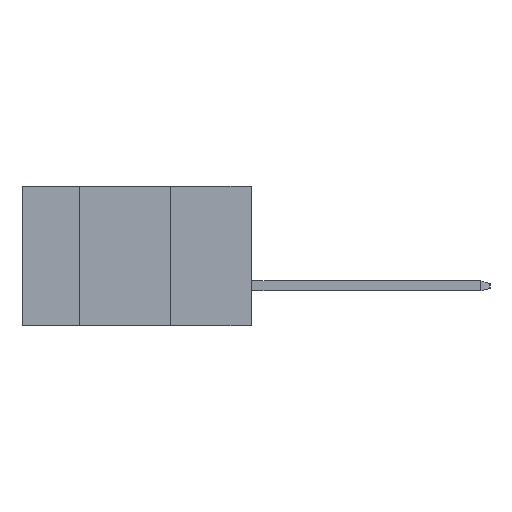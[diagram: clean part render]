
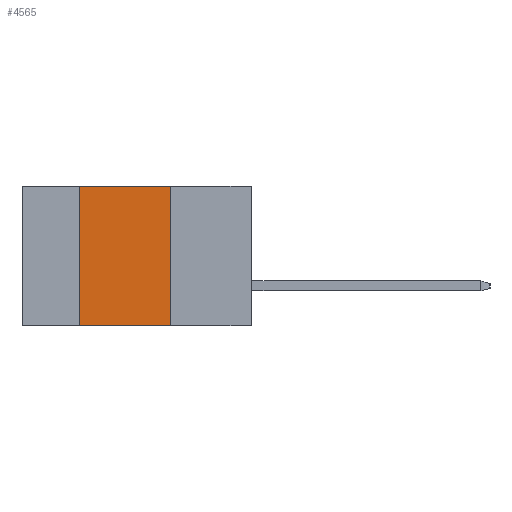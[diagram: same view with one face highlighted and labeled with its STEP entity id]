
A CAD part, left-side view. The second image highlights one B-rep face of the part: STEP entity #4565.
In plain terms, the highlighted planar face has unit normal (-1, 0, 0).
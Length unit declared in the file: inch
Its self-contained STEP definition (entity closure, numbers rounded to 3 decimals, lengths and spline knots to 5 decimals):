
#315 = EDGE_CURVE ( 'NONE', #5962, #707, #1120, .T. ) ;
#588 = CARTESIAN_POINT ( 'NONE',  ( 0., 0.54, -0.437 ) ) ;
#688 = CARTESIAN_POINT ( 'NONE',  ( 0., 0.72, 0. ) ) ;
#707 = VERTEX_POINT ( 'NONE', #6120 ) ;
#947 = ORIENTED_EDGE ( 'NONE', *, *, #7936, .T. ) ;
#1120 = LINE ( 'NONE', #6609, #1316 ) ;
#1316 = VECTOR ( 'NONE', #9772, 39.37008 ) ;
#1499 = ORIENTED_EDGE ( 'NONE', *, *, #315, .F. ) ;
#1582 = EDGE_LOOP ( 'NONE', ( #1499, #2919, #4034, #947 ) ) ;
#2122 = FACE_OUTER_BOUND ( 'NONE', #1582, .T. ) ;
#2214 = VECTOR ( 'NONE', #7254, 39.37008 ) ;
#2231 = DIRECTION ( 'NONE',  ( 1., 0., 0. ) ) ;
#2919 = ORIENTED_EDGE ( 'NONE', *, *, #5681, .F. ) ;
#3491 = AXIS2_PLACEMENT_3D ( 'NONE', #688, #2231, #10008 ) ;
#3810 = DIRECTION ( 'NONE',  ( 0., 0., 1. ) ) ;
#3975 = VERTEX_POINT ( 'NONE', #6569 ) ;
#4034 = ORIENTED_EDGE ( 'NONE', *, *, #6354, .F. ) ;
#4361 = CARTESIAN_POINT ( 'NONE',  ( 0., 0.72, -0.437 ) ) ;
#4501 = CARTESIAN_POINT ( 'NONE',  ( 0., 0.254, 0. ) ) ;
#4565 = ADVANCED_FACE ( 'NONE', ( #2122 ), #8394, .F. ) ;
#4643 = VECTOR ( 'NONE', #8728, 39.37008 ) ;
#4824 = CARTESIAN_POINT ( 'NONE',  ( 0., 0.72, 0. ) ) ;
#5681 = EDGE_CURVE ( 'NONE', #7654, #5962, #8578, .T. ) ;
#5962 = VERTEX_POINT ( 'NONE', #4501 ) ;
#6120 = CARTESIAN_POINT ( 'NONE',  ( 0., 0.254, -0.437 ) ) ;
#6190 = LINE ( 'NONE', #4361, #2214 ) ;
#6354 = EDGE_CURVE ( 'NONE', #3975, #7654, #9272, .T. ) ;
#6569 = CARTESIAN_POINT ( 'NONE',  ( 0., 0.54, -0.437 ) ) ;
#6609 = CARTESIAN_POINT ( 'NONE',  ( 0., 0.254, -0.437 ) ) ;
#7254 = DIRECTION ( 'NONE',  ( 0., -1., 0. ) ) ;
#7654 = VERTEX_POINT ( 'NONE', #8247 ) ;
#7936 = EDGE_CURVE ( 'NONE', #3975, #707, #6190, .T. ) ;
#8247 = CARTESIAN_POINT ( 'NONE',  ( 0., 0.54, 0. ) ) ;
#8394 = PLANE ( 'NONE',  #3491 ) ;
#8578 = LINE ( 'NONE', #4824, #4643 ) ;
#8728 = DIRECTION ( 'NONE',  ( 0., -1., 0. ) ) ;
#9272 = LINE ( 'NONE', #588, #9422 ) ;
#9422 = VECTOR ( 'NONE', #3810, 39.37008 ) ;
#9772 = DIRECTION ( 'NONE',  ( 0., 0., -1. ) ) ;
#10008 = DIRECTION ( 'NONE',  ( 0., 0., -1. ) ) ;
